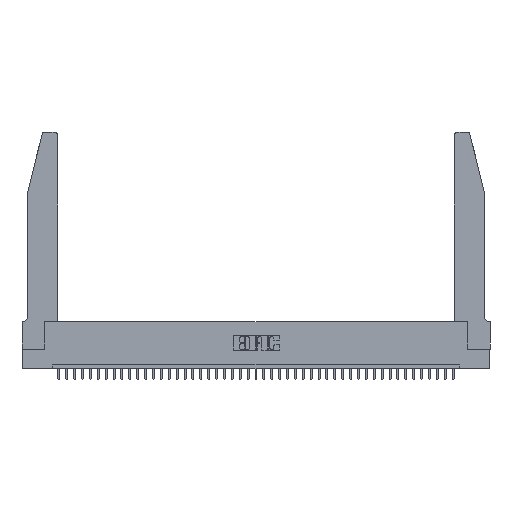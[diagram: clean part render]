
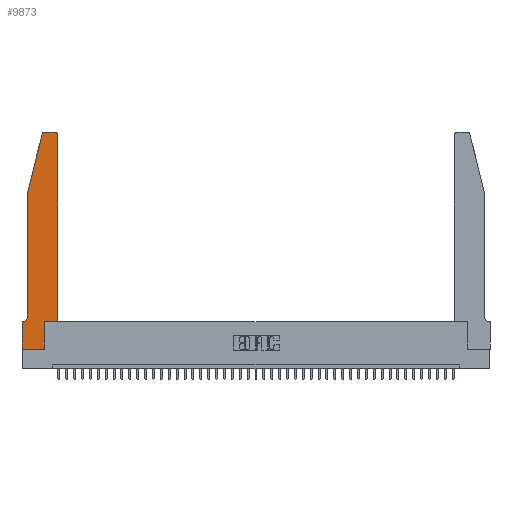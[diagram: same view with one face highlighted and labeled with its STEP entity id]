
A CAD part, top view. The second image highlights one B-rep face of the part: STEP entity #9873.
In plain terms, the highlighted planar face has unit normal (0, 0, 1).
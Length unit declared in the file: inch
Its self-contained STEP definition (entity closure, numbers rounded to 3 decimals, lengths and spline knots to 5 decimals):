
#379 = DIRECTION ( 'NONE',  ( 1., 0., 0. ) ) ;
#772 = ORIENTED_EDGE ( 'NONE', *, *, #38826, .T. ) ;
#1338 = DIRECTION ( 'NONE',  ( 0., 0., 1. ) ) ;
#2875 = ORIENTED_EDGE ( 'NONE', *, *, #35629, .T. ) ;
#2970 = VERTEX_POINT ( 'NONE', #22930 ) ;
#3112 = EDGE_CURVE ( 'NONE', #3527, #41952, #28235, .T. ) ;
#3214 = LINE ( 'NONE', #8555, #16357 ) ;
#3357 = VERTEX_POINT ( 'NONE', #17042 ) ;
#3527 = VERTEX_POINT ( 'NONE', #14334 ) ;
#4103 = EDGE_CURVE ( 'NONE', #11685, #20002, #8334, .T. ) ;
#4187 = CARTESIAN_POINT ( 'NONE',  ( 0., 0., 0.37 ) ) ;
#4889 = CARTESIAN_POINT ( 'NONE',  ( 0.4505, 0.35, 0.37 ) ) ;
#5323 = VECTOR ( 'NONE', #30403, 39.37008 ) ;
#5423 = ORIENTED_EDGE ( 'NONE', *, *, #4103, .T. ) ;
#5783 = DIRECTION ( 'NONE',  ( -1., 0., 0. ) ) ;
#6345 = PLANE ( 'NONE',  #28053 ) ;
#6540 = DIRECTION ( 'NONE',  ( 1., 0., 0. ) ) ;
#7113 = CARTESIAN_POINT ( 'NONE',  ( 0.2865, 0.35, 0.37 ) ) ;
#7686 = ORIENTED_EDGE ( 'NONE', *, *, #22530, .T. ) ;
#8334 = LINE ( 'NONE', #41138, #29113 ) ;
#8555 = CARTESIAN_POINT ( 'NONE',  ( 0., 0., 0.37 ) ) ;
#9056 = AXIS2_PLACEMENT_3D ( 'NONE', #11751, #30691, #14381 ) ;
#9873 = ADVANCED_FACE ( 'NONE', ( #10462 ), #6345, .T. ) ;
#10462 = FACE_OUTER_BOUND ( 'NONE', #29588, .T. ) ;
#10706 = AXIS2_PLACEMENT_3D ( 'NONE', #17490, #1338, #24024 ) ;
#10850 = ORIENTED_EDGE ( 'NONE', *, *, #35022, .T. ) ;
#10899 = CARTESIAN_POINT ( 'NONE',  ( 0.2605, 2.75, 0.37 ) ) ;
#10917 = VECTOR ( 'NONE', #40316, 39.37008 ) ;
#11244 = CARTESIAN_POINT ( 'NONE',  ( 0., 0., 0.37 ) ) ;
#11538 = LINE ( 'NONE', #10899, #16096 ) ;
#11685 = VERTEX_POINT ( 'NONE', #12806 ) ;
#11751 = CARTESIAN_POINT ( 'NONE',  ( 0.284, 2.72, 0.37 ) ) ;
#12806 = CARTESIAN_POINT ( 'NONE',  ( 0.0055, 0.35, 0.37 ) ) ;
#13451 = ORIENTED_EDGE ( 'NONE', *, *, #39026, .T. ) ;
#14334 = CARTESIAN_POINT ( 'NONE',  ( 0.2865, 0., 0.37 ) ) ;
#14381 = DIRECTION ( 'NONE',  ( 1., 0., 0. ) ) ;
#14937 = VECTOR ( 'NONE', #27573, 39.37008 ) ;
#15698 = CARTESIAN_POINT ( 'NONE',  ( 0.4505, 2.72, 0.37 ) ) ;
#15984 = LINE ( 'NONE', #4889, #14937 ) ;
#16083 = CARTESIAN_POINT ( 'NONE',  ( 0., 0.35, 0.37 ) ) ;
#16096 = VECTOR ( 'NONE', #36618, 39.37008 ) ;
#16357 = VECTOR ( 'NONE', #379, 39.37008 ) ;
#16748 = EDGE_CURVE ( 'NONE', #41952, #26716, #35647, .T. ) ;
#17042 = CARTESIAN_POINT ( 'NONE',  ( 0.4205, 2.75, 0.37 ) ) ;
#17490 = CARTESIAN_POINT ( 'NONE',  ( 0.4205, 2.72, 0.37 ) ) ;
#18118 = CIRCLE ( 'NONE', #9056, 0.03 ) ;
#18238 = DIRECTION ( 'NONE',  ( 0., -1., 0. ) ) ;
#18573 = EDGE_CURVE ( 'NONE', #2970, #29691, #22597, .T. ) ;
#20002 = VERTEX_POINT ( 'NONE', #30325 ) ;
#20549 = ORIENTED_EDGE ( 'NONE', *, *, #40737, .T. ) ;
#20676 = CIRCLE ( 'NONE', #25443, 0.07 ) ;
#22105 = DIRECTION ( 'NONE',  ( 0., 0., -1. ) ) ;
#22308 = CIRCLE ( 'NONE', #10706, 0.03 ) ;
#22530 = EDGE_CURVE ( 'NONE', #27099, #2970, #18118, .T. ) ;
#22597 = LINE ( 'NONE', #39709, #5323 ) ;
#22930 = CARTESIAN_POINT ( 'NONE',  ( 0.25487, 2.72718, 0.37 ) ) ;
#23636 = VECTOR ( 'NONE', #36710, 39.37008 ) ;
#23754 = CARTESIAN_POINT ( 'NONE',  ( 0.2865, 0.35, 0.37 ) ) ;
#23836 = ORIENTED_EDGE ( 'NONE', *, *, #31430, .T. ) ;
#24024 = DIRECTION ( 'NONE',  ( 1., 0., 0. ) ) ;
#25051 = DIRECTION ( 'NONE',  ( -1., 0., 0. ) ) ;
#25136 = CARTESIAN_POINT ( 'NONE',  ( 0.284, 2.75, 0.37 ) ) ;
#25443 = AXIS2_PLACEMENT_3D ( 'NONE', #38140, #22105, #25051 ) ;
#26408 = DIRECTION ( 'NONE',  ( 0., 0., 1. ) ) ;
#26716 = VERTEX_POINT ( 'NONE', #41262 ) ;
#27099 = VERTEX_POINT ( 'NONE', #25136 ) ;
#27573 = DIRECTION ( 'NONE',  ( 0., 1., 0. ) ) ;
#27893 = ORIENTED_EDGE ( 'NONE', *, *, #3112, .T. ) ;
#28053 = AXIS2_PLACEMENT_3D ( 'NONE', #16083, #26408, #6540 ) ;
#28235 = LINE ( 'NONE', #7113, #10917 ) ;
#28319 = ORIENTED_EDGE ( 'NONE', *, *, #16748, .T. ) ;
#28336 = CARTESIAN_POINT ( 'NONE',  ( 0.0755, 0.42, 0.37 ) ) ;
#29036 = ORIENTED_EDGE ( 'NONE', *, *, #18573, .T. ) ;
#29113 = VECTOR ( 'NONE', #5783, 39.37008 ) ;
#29341 = VECTOR ( 'NONE', #18238, 39.37008 ) ;
#29588 = EDGE_LOOP ( 'NONE', ( #10850, #7686, #29036, #772, #13451, #5423, #2875, #23836, #27893, #28319, #20549, #30756 ) ) ;
#29691 = VERTEX_POINT ( 'NONE', #32665 ) ;
#30293 = LINE ( 'NONE', #40414, #29341 ) ;
#30325 = CARTESIAN_POINT ( 'NONE',  ( 0., 0.35, 0.37 ) ) ;
#30403 = DIRECTION ( 'NONE',  ( -0.239, -0.971, 0. ) ) ;
#30691 = DIRECTION ( 'NONE',  ( 0., 0., 1. ) ) ;
#30756 = ORIENTED_EDGE ( 'NONE', *, *, #38777, .T. ) ;
#30796 = VERTEX_POINT ( 'NONE', #15698 ) ;
#31430 = EDGE_CURVE ( 'NONE', #36243, #3527, #3214, .T. ) ;
#32665 = CARTESIAN_POINT ( 'NONE',  ( 0.0755, 2., 0.37 ) ) ;
#35022 = EDGE_CURVE ( 'NONE', #3357, #27099, #11538, .T. ) ;
#35360 = CARTESIAN_POINT ( 'NONE',  ( 0.4505, 0.35, 0.37 ) ) ;
#35629 = EDGE_CURVE ( 'NONE', #20002, #36243, #37808, .T. ) ;
#35647 = LINE ( 'NONE', #35360, #40765 ) ;
#35850 = VERTEX_POINT ( 'NONE', #28336 ) ;
#36243 = VERTEX_POINT ( 'NONE', #11244 ) ;
#36618 = DIRECTION ( 'NONE',  ( -1., 0., 0. ) ) ;
#36689 = DIRECTION ( 'NONE',  ( 1., 0., 0. ) ) ;
#36710 = DIRECTION ( 'NONE',  ( 0., -1., 0. ) ) ;
#37808 = LINE ( 'NONE', #4187, #23636 ) ;
#38140 = CARTESIAN_POINT ( 'NONE',  ( 0.0055, 0.42, 0.37 ) ) ;
#38777 = EDGE_CURVE ( 'NONE', #30796, #3357, #22308, .T. ) ;
#38826 = EDGE_CURVE ( 'NONE', #29691, #35850, #30293, .T. ) ;
#39026 = EDGE_CURVE ( 'NONE', #35850, #11685, #20676, .T. ) ;
#39709 = CARTESIAN_POINT ( 'NONE',  ( 0.0755, 2., 0.37 ) ) ;
#40316 = DIRECTION ( 'NONE',  ( 0., 1., 0. ) ) ;
#40414 = CARTESIAN_POINT ( 'NONE',  ( 0.0755, 2., 0.37 ) ) ;
#40737 = EDGE_CURVE ( 'NONE', #26716, #30796, #15984, .T. ) ;
#40765 = VECTOR ( 'NONE', #36689, 39.37008 ) ;
#41138 = CARTESIAN_POINT ( 'NONE',  ( 0.0755, 0.35, 0.37 ) ) ;
#41262 = CARTESIAN_POINT ( 'NONE',  ( 0.4505, 0.35, 0.37 ) ) ;
#41952 = VERTEX_POINT ( 'NONE', #23754 ) ;
